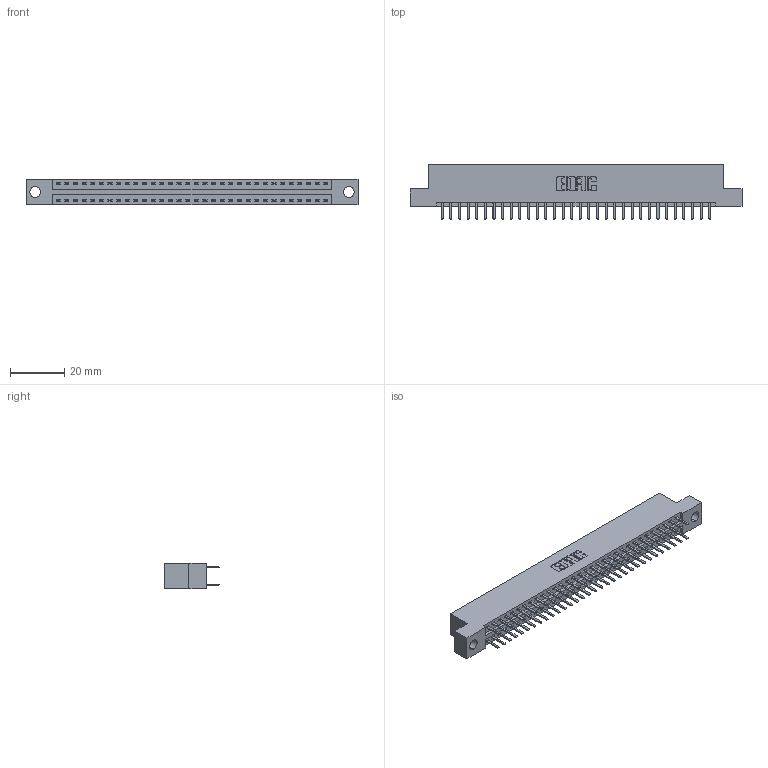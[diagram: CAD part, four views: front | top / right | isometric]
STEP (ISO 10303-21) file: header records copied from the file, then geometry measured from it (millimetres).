
FILE_DESCRIPTION (( 'STEP AP203' ), '1' );
FILE_NAME ('346-064-520-204.STEP', '2022-05-24T14:51:16', ( '' ), ( '' ), 'SwSTEP 2.0', 'SolidWorks 2020', '' );
FILE_SCHEMA (( 'CONFIG_CONTROL_DESIGN' ));
Length unit declared in the file: inch
Products named in the file (3): 345-292-001_345-293-120; 346 Part_Flush Mounting Lugs - 0.156 Dia-TH; 346-064-520-204
Assembly tree (65 placements, depth 2):
  346-064-520-204
    346 Part_Flush Mounting Lugs - 0.156 Dia-TH
    345-292-001_345-293-120  x64
Bounding box: 122.17 x 20.02 x 9.4 mm (x, y, z)
Volume: 11701.7 mm3; surface area: 15709.6 mm2
Topology: 65 solids, 65 shells, 3720 faces, 10797 edges, 7026 vertices
Faces by surface type: plane 2458, cylinder 1262
Entity records: 22763 total; most frequent: CARTESIAN_POINT 3782, ORIENTED_EDGE 3702, DIRECTION 3371, EDGE_CURVE 1851, LINE 1587, VECTOR 1587, VERTEX_POINT 1230, AXIS2_PLACEMENT_3D 892
